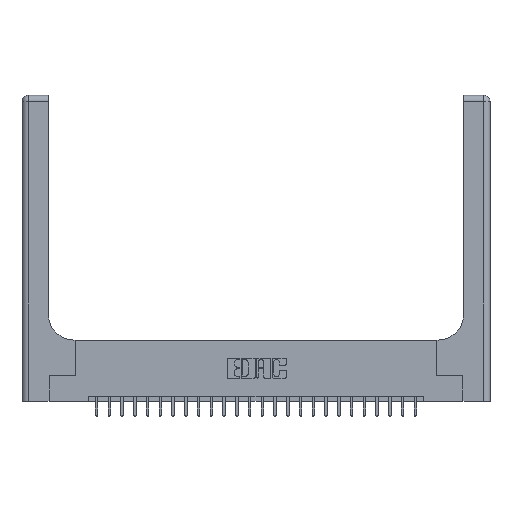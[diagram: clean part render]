
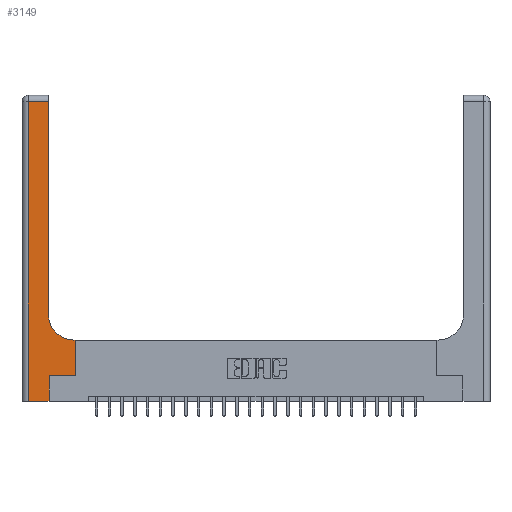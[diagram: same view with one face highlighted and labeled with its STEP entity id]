
A CAD part, top view. The second image highlights one B-rep face of the part: STEP entity #3149.
In plain terms, the highlighted planar face has unit normal (0, 0, 1).
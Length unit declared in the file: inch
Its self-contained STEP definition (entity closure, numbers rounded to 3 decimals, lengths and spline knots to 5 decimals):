
#61 = CARTESIAN_POINT ( 'NONE',  ( 0.265, 0.25, 0.37 ) ) ;
#701 = VECTOR ( 'NONE', #1631, 39.37008 ) ;
#852 = EDGE_CURVE ( 'NONE', #17839, #6176, #7979, .T. ) ;
#868 = VECTOR ( 'NONE', #11092, 39.37008 ) ;
#996 = CARTESIAN_POINT ( 'NONE',  ( 0.51, 0.6, 0.37 ) ) ;
#997 = ORIENTED_EDGE ( 'NONE', *, *, #852, .T. ) ;
#1299 = LINE ( 'NONE', #18342, #701 ) ;
#1631 = DIRECTION ( 'NONE',  ( 0., 1., 0. ) ) ;
#1676 = CARTESIAN_POINT ( 'NONE',  ( 0.26, 3., 0.37 ) ) ;
#2104 = CARTESIAN_POINT ( 'NONE',  ( 0.528, 0.25, 0.37 ) ) ;
#2205 = ORIENTED_EDGE ( 'NONE', *, *, #15581, .T. ) ;
#2609 = CARTESIAN_POINT ( 'NONE',  ( 0.528, 0.25, 0.37 ) ) ;
#2623 = CARTESIAN_POINT ( 'NONE',  ( 0.26, 2.94, 0.37 ) ) ;
#2778 = ORIENTED_EDGE ( 'NONE', *, *, #9738, .T. ) ;
#3149 = ADVANCED_FACE ( 'NONE', ( #21926 ), #24050, .F. ) ;
#3449 = CARTESIAN_POINT ( 'NONE',  ( 0.265, 0.25, 0.37 ) ) ;
#3472 = DIRECTION ( 'NONE',  ( -1., 0., 0. ) ) ;
#3939 = LINE ( 'NONE', #2104, #14543 ) ;
#4200 = CARTESIAN_POINT ( 'NONE',  ( 0.51, 0.85, 0.37 ) ) ;
#4379 = DIRECTION ( 'NONE',  ( 1., 0., 0. ) ) ;
#4456 = VECTOR ( 'NONE', #10423, 39.37008 ) ;
#4702 = VERTEX_POINT ( 'NONE', #2623 ) ;
#5230 = ORIENTED_EDGE ( 'NONE', *, *, #14595, .T. ) ;
#5241 = LINE ( 'NONE', #12096, #18712 ) ;
#5439 = VERTEX_POINT ( 'NONE', #996 ) ;
#5781 = VECTOR ( 'NONE', #13925, 39.37008 ) ;
#5820 = DIRECTION ( 'NONE',  ( 0., 1., 0. ) ) ;
#5948 = CARTESIAN_POINT ( 'NONE',  ( 0., 3., 0.37 ) ) ;
#6176 = VERTEX_POINT ( 'NONE', #6762 ) ;
#6404 = LINE ( 'NONE', #1676, #6684 ) ;
#6684 = VECTOR ( 'NONE', #5820, 39.37008 ) ;
#6762 = CARTESIAN_POINT ( 'NONE',  ( 0.265, 0., 0.37 ) ) ;
#7501 = CARTESIAN_POINT ( 'NONE',  ( 0.06, 3., 0.37 ) ) ;
#7979 = LINE ( 'NONE', #19730, #4456 ) ;
#8201 = CARTESIAN_POINT ( 'NONE',  ( 0., 2.94, 0.37 ) ) ;
#8416 = VERTEX_POINT ( 'NONE', #2609 ) ;
#8696 = ORIENTED_EDGE ( 'NONE', *, *, #22145, .T. ) ;
#9679 = LINE ( 'NONE', #7501, #11746 ) ;
#9738 = EDGE_CURVE ( 'NONE', #11896, #5439, #5241, .T. ) ;
#9789 = CARTESIAN_POINT ( 'NONE',  ( 0.06, 0., 0.37 ) ) ;
#9980 = VERTEX_POINT ( 'NONE', #18256 ) ;
#10070 = CARTESIAN_POINT ( 'NONE',  ( 0.26, 0.85, 0.37 ) ) ;
#10423 = DIRECTION ( 'NONE',  ( 1., 0., 0. ) ) ;
#11092 = DIRECTION ( 'NONE',  ( 1., 0., 0. ) ) ;
#11100 = ORIENTED_EDGE ( 'NONE', *, *, #23208, .T. ) ;
#11746 = VECTOR ( 'NONE', #20574, 39.37008 ) ;
#11896 = VERTEX_POINT ( 'NONE', #23148 ) ;
#12096 = CARTESIAN_POINT ( 'NONE',  ( 0.26, 0.6, 0.37 ) ) ;
#12815 = DIRECTION ( 'NONE',  ( 0., 0., -1. ) ) ;
#13357 = EDGE_CURVE ( 'NONE', #16672, #4702, #6404, .T. ) ;
#13374 = ORIENTED_EDGE ( 'NONE', *, *, #18249, .T. ) ;
#13593 = DIRECTION ( 'NONE',  ( 0., 1., 0. ) ) ;
#13813 = DIRECTION ( 'NONE',  ( 0., 0., -1. ) ) ;
#13925 = DIRECTION ( 'NONE',  ( -1., 0., 0. ) ) ;
#14543 = VECTOR ( 'NONE', #13593, 39.37008 ) ;
#14595 = EDGE_CURVE ( 'NONE', #4702, #9980, #23667, .T. ) ;
#15044 = VERTEX_POINT ( 'NONE', #61 ) ;
#15581 = EDGE_CURVE ( 'NONE', #6176, #15044, #1299, .T. ) ;
#16107 = ORIENTED_EDGE ( 'NONE', *, *, #19620, .T. ) ;
#16239 = CIRCLE ( 'NONE', #23430, 0.25 ) ;
#16672 = VERTEX_POINT ( 'NONE', #10070 ) ;
#17839 = VERTEX_POINT ( 'NONE', #9789 ) ;
#18249 = EDGE_CURVE ( 'NONE', #15044, #8416, #24072, .T. ) ;
#18256 = CARTESIAN_POINT ( 'NONE',  ( 0.06, 2.94, 0.37 ) ) ;
#18342 = CARTESIAN_POINT ( 'NONE',  ( 0.265, 0., 0.37 ) ) ;
#18712 = VECTOR ( 'NONE', #21228, 39.37008 ) ;
#19620 = EDGE_CURVE ( 'NONE', #9980, #17839, #9679, .T. ) ;
#19730 = CARTESIAN_POINT ( 'NONE',  ( 0., 0., 0.37 ) ) ;
#20574 = DIRECTION ( 'NONE',  ( 0., -1., 0. ) ) ;
#21228 = DIRECTION ( 'NONE',  ( -1., 0., 0. ) ) ;
#21331 = ORIENTED_EDGE ( 'NONE', *, *, #13357, .T. ) ;
#21926 = FACE_OUTER_BOUND ( 'NONE', #22043, .T. ) ;
#22043 = EDGE_LOOP ( 'NONE', ( #21331, #5230, #16107, #997, #2205, #13374, #8696, #2778, #11100 ) ) ;
#22145 = EDGE_CURVE ( 'NONE', #8416, #11896, #3939, .T. ) ;
#23148 = CARTESIAN_POINT ( 'NONE',  ( 0.528, 0.6, 0.37 ) ) ;
#23208 = EDGE_CURVE ( 'NONE', #5439, #16672, #16239, .T. ) ;
#23249 = AXIS2_PLACEMENT_3D ( 'NONE', #5948, #12815, #3472 ) ;
#23430 = AXIS2_PLACEMENT_3D ( 'NONE', #4200, #13813, #4379 ) ;
#23667 = LINE ( 'NONE', #8201, #5781 ) ;
#24050 = PLANE ( 'NONE',  #23249 ) ;
#24072 = LINE ( 'NONE', #3449, #868 ) ;
